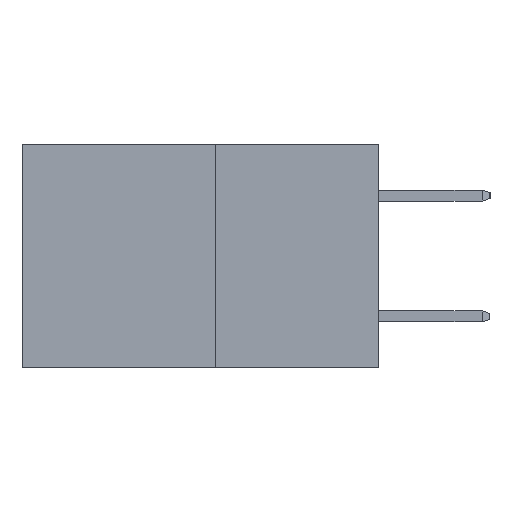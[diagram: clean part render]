
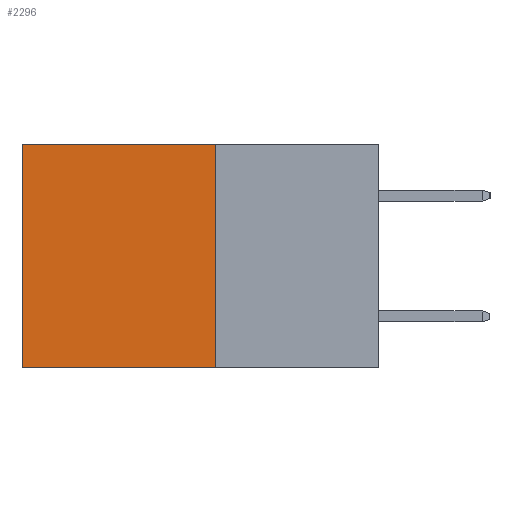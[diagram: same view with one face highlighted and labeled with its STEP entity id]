
A CAD part, left-side view. The second image highlights one B-rep face of the part: STEP entity #2296.
In plain terms, the highlighted planar face has unit normal (-1, 0, 0).
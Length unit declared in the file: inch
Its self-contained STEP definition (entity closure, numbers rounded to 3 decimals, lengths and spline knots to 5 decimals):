
#755 = VERTEX_POINT ( 'NONE', #11857 ) ;
#813 = EDGE_CURVE ( 'NONE', #2826, #755, #15701, .T. ) ;
#1821 = VECTOR ( 'NONE', #8261, 39.37008 ) ;
#1922 = EDGE_CURVE ( 'NONE', #14964, #16339, #12367, .T. ) ;
#2124 = EDGE_LOOP ( 'NONE', ( #4797, #5381, #5736, #5987 ) ) ;
#2252 = DIRECTION ( 'NONE',  ( 0., 1., 0. ) ) ;
#2296 = ADVANCED_FACE ( 'NONE', ( #7482 ), #13891, .F. ) ;
#2376 = DIRECTION ( 'NONE',  ( 0., 0., -1. ) ) ;
#2826 = VERTEX_POINT ( 'NONE', #5161 ) ;
#3283 = DIRECTION ( 'NONE',  ( 0., 0., -1. ) ) ;
#4355 = CARTESIAN_POINT ( 'NONE',  ( 0.277, 0.59, 0. ) ) ;
#4797 = ORIENTED_EDGE ( 'NONE', *, *, #11095, .T. ) ;
#5161 = CARTESIAN_POINT ( 'NONE',  ( 0.277, 0.27, -0.37 ) ) ;
#5381 = ORIENTED_EDGE ( 'NONE', *, *, #813, .F. ) ;
#5736 = ORIENTED_EDGE ( 'NONE', *, *, #6811, .F. ) ;
#5976 = VECTOR ( 'NONE', #2376, 39.37008 ) ;
#5987 = ORIENTED_EDGE ( 'NONE', *, *, #1922, .T. ) ;
#6028 = DIRECTION ( 'NONE',  ( 0., 0., -1. ) ) ;
#6811 = EDGE_CURVE ( 'NONE', #14964, #2826, #16406, .T. ) ;
#7417 = CARTESIAN_POINT ( 'NONE',  ( 0.277, 0.27, 0. ) ) ;
#7482 = FACE_OUTER_BOUND ( 'NONE', #2124, .T. ) ;
#8261 = DIRECTION ( 'NONE',  ( 0., 1., 0. ) ) ;
#9237 = CARTESIAN_POINT ( 'NONE',  ( 0.277, 0.27, -0.37 ) ) ;
#9543 = DIRECTION ( 'NONE',  ( 1., 0., 0. ) ) ;
#10652 = CARTESIAN_POINT ( 'NONE',  ( 0.277, 0.27, -0.37 ) ) ;
#11095 = EDGE_CURVE ( 'NONE', #16339, #755, #14337, .T. ) ;
#11389 = CARTESIAN_POINT ( 'NONE',  ( 0.277, 0.27, -0.37 ) ) ;
#11857 = CARTESIAN_POINT ( 'NONE',  ( 0.277, 0.59, -0.37 ) ) ;
#12033 = VECTOR ( 'NONE', #2252, 39.37008 ) ;
#12367 = LINE ( 'NONE', #13759, #1821 ) ;
#12771 = CARTESIAN_POINT ( 'NONE',  ( 0.277, 0.59, -0.37 ) ) ;
#13759 = CARTESIAN_POINT ( 'NONE',  ( 0.277, 0.27, 0. ) ) ;
#13891 = PLANE ( 'NONE',  #14055 ) ;
#14055 = AXIS2_PLACEMENT_3D ( 'NONE', #9237, #9543, #3283 ) ;
#14337 = LINE ( 'NONE', #12771, #17463 ) ;
#14964 = VERTEX_POINT ( 'NONE', #7417 ) ;
#15701 = LINE ( 'NONE', #11389, #12033 ) ;
#16339 = VERTEX_POINT ( 'NONE', #4355 ) ;
#16406 = LINE ( 'NONE', #10652, #5976 ) ;
#17463 = VECTOR ( 'NONE', #6028, 39.37008 ) ;
